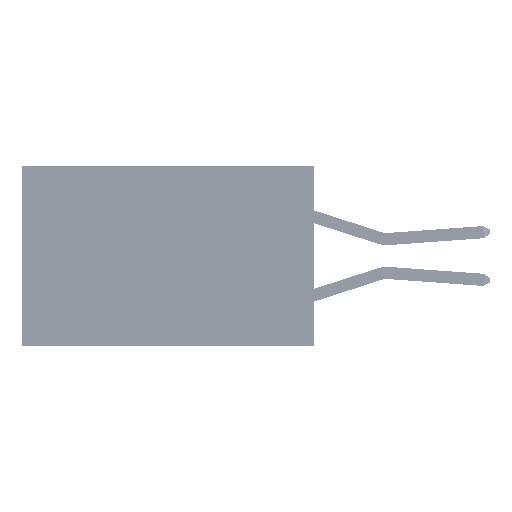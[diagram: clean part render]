
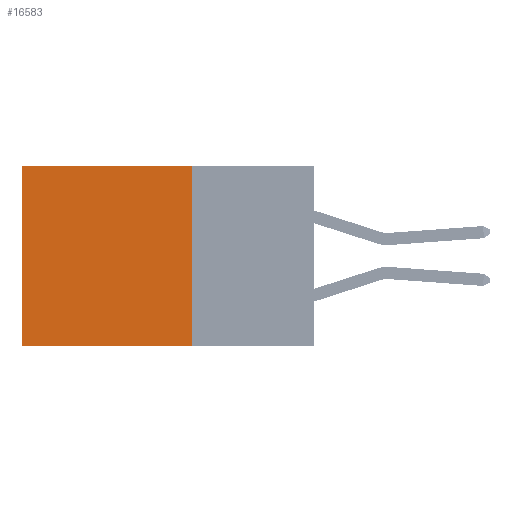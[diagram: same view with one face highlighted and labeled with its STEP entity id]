
A CAD part, left-side view. The second image highlights one B-rep face of the part: STEP entity #16583.
In plain terms, the highlighted planar face has unit normal (-1, 0, 0).
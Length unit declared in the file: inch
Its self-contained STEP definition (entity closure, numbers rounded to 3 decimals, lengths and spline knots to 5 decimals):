
#172 = EDGE_CURVE ( 'NONE', #6090, #34474, #9251, .T. ) ;
#718 = DIRECTION ( 'NONE',  ( 0., 0., -1. ) ) ;
#1255 = LINE ( 'NONE', #19805, #15822 ) ;
#1294 = FACE_OUTER_BOUND ( 'NONE', #24211, .T. ) ;
#2724 = VECTOR ( 'NONE', #39832, 39.37008 ) ;
#3121 = EDGE_CURVE ( 'NONE', #22981, #22033, #32164, .T. ) ;
#5762 = DIRECTION ( 'NONE',  ( 0., 1., 0. ) ) ;
#5828 = CARTESIAN_POINT ( 'NONE',  ( 0.2875, 0.25, 0. ) ) ;
#6090 = VERTEX_POINT ( 'NONE', #5828 ) ;
#9251 = LINE ( 'NONE', #43364, #38614 ) ;
#11425 = DIRECTION ( 'NONE',  ( 1., 0., 0. ) ) ;
#12384 = ORIENTED_EDGE ( 'NONE', *, *, #33135, .T. ) ;
#15822 = VECTOR ( 'NONE', #5762, 39.37008 ) ;
#15994 = LINE ( 'NONE', #24078, #43655 ) ;
#16583 = ADVANCED_FACE ( 'NONE', ( #1294 ), #37793, .F. ) ;
#19805 = CARTESIAN_POINT ( 'NONE',  ( 0.2875, 0.25, -0.37 ) ) ;
#20497 = EDGE_CURVE ( 'NONE', #34474, #22033, #1255, .T. ) ;
#22033 = VERTEX_POINT ( 'NONE', #39415 ) ;
#22981 = VERTEX_POINT ( 'NONE', #36161 ) ;
#24078 = CARTESIAN_POINT ( 'NONE',  ( 0.2875, 0.25, 0. ) ) ;
#24211 = EDGE_LOOP ( 'NONE', ( #28928, #37195, #38210, #12384 ) ) ;
#27417 = AXIS2_PLACEMENT_3D ( 'NONE', #33098, #11425, #718 ) ;
#28928 = ORIENTED_EDGE ( 'NONE', *, *, #3121, .T. ) ;
#32164 = LINE ( 'NONE', #40134, #2724 ) ;
#32512 = DIRECTION ( 'NONE',  ( 0., 0., -1. ) ) ;
#33098 = CARTESIAN_POINT ( 'NONE',  ( 0.2875, 0.25, 0. ) ) ;
#33135 = EDGE_CURVE ( 'NONE', #6090, #22981, #15994, .T. ) ;
#34474 = VERTEX_POINT ( 'NONE', #38787 ) ;
#36161 = CARTESIAN_POINT ( 'NONE',  ( 0.2875, 0.6, 0. ) ) ;
#37195 = ORIENTED_EDGE ( 'NONE', *, *, #20497, .F. ) ;
#37793 = PLANE ( 'NONE',  #27417 ) ;
#38210 = ORIENTED_EDGE ( 'NONE', *, *, #172, .F. ) ;
#38614 = VECTOR ( 'NONE', #32512, 39.37008 ) ;
#38787 = CARTESIAN_POINT ( 'NONE',  ( 0.2875, 0.25, -0.37 ) ) ;
#39415 = CARTESIAN_POINT ( 'NONE',  ( 0.2875, 0.6, -0.37 ) ) ;
#39832 = DIRECTION ( 'NONE',  ( 0., 0., -1. ) ) ;
#40134 = CARTESIAN_POINT ( 'NONE',  ( 0.2875, 0.6, 0. ) ) ;
#42368 = DIRECTION ( 'NONE',  ( 0., 1., 0. ) ) ;
#43364 = CARTESIAN_POINT ( 'NONE',  ( 0.2875, 0.25, 0. ) ) ;
#43655 = VECTOR ( 'NONE', #42368, 39.37008 ) ;
